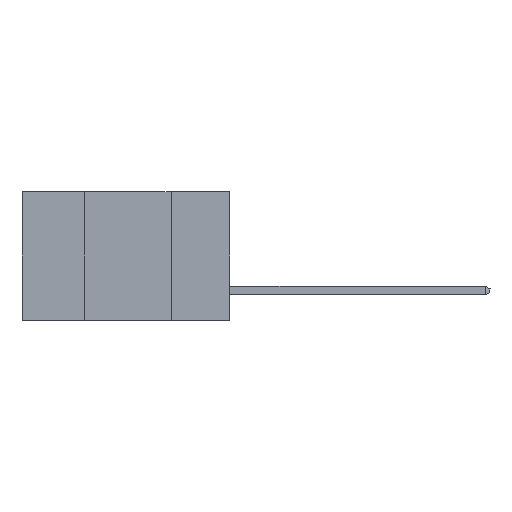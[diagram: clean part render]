
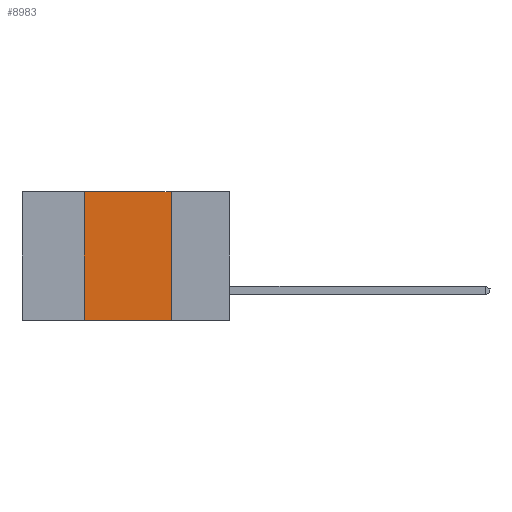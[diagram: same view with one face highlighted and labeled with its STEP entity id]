
A CAD part, left-side view. The second image highlights one B-rep face of the part: STEP entity #8983.
In plain terms, the highlighted planar face has unit normal (-1, 0, 0).
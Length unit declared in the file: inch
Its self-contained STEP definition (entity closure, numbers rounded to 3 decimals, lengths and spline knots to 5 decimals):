
#184 = VERTEX_POINT ( 'NONE', #4836 ) ;
#264 = EDGE_CURVE ( 'NONE', #184, #1446, #3708, .T. ) ;
#720 = DIRECTION ( 'NONE',  ( 0., -1., 0. ) ) ;
#741 = LINE ( 'NONE', #7236, #4051 ) ;
#1446 = VERTEX_POINT ( 'NONE', #8938 ) ;
#1547 = CARTESIAN_POINT ( 'NONE',  ( 0., 0.6, -0.37 ) ) ;
#1563 = VECTOR ( 'NONE', #4553, 39.37008 ) ;
#1700 = LINE ( 'NONE', #7397, #1563 ) ;
#1803 = DIRECTION ( 'NONE',  ( 1., 0., 0. ) ) ;
#2610 = ORIENTED_EDGE ( 'NONE', *, *, #6053, .F. ) ;
#2784 = VERTEX_POINT ( 'NONE', #3439 ) ;
#3439 = CARTESIAN_POINT ( 'NONE',  ( 0., 0.17, 0. ) ) ;
#3491 = CARTESIAN_POINT ( 'NONE',  ( 0., 0.6, 0. ) ) ;
#3534 = VECTOR ( 'NONE', #7159, 39.37008 ) ;
#3708 = LINE ( 'NONE', #1547, #3534 ) ;
#3890 = CARTESIAN_POINT ( 'NONE',  ( 0., 0.42, 0. ) ) ;
#4051 = VECTOR ( 'NONE', #8603, 39.37008 ) ;
#4087 = EDGE_CURVE ( 'NONE', #2784, #1446, #1700, .T. ) ;
#4553 = DIRECTION ( 'NONE',  ( 0., 0., -1. ) ) ;
#4580 = AXIS2_PLACEMENT_3D ( 'NONE', #4656, #1803, #5968 ) ;
#4656 = CARTESIAN_POINT ( 'NONE',  ( 0., 0.6, 0. ) ) ;
#4836 = CARTESIAN_POINT ( 'NONE',  ( 0., 0.42, -0.37 ) ) ;
#5589 = LINE ( 'NONE', #3491, #6911 ) ;
#5658 = ORIENTED_EDGE ( 'NONE', *, *, #6876, .F. ) ;
#5968 = DIRECTION ( 'NONE',  ( 0., 0., -1. ) ) ;
#6053 = EDGE_CURVE ( 'NONE', #184, #7036, #741, .T. ) ;
#6180 = ORIENTED_EDGE ( 'NONE', *, *, #4087, .F. ) ;
#6804 = EDGE_LOOP ( 'NONE', ( #6180, #5658, #2610, #8235 ) ) ;
#6876 = EDGE_CURVE ( 'NONE', #7036, #2784, #5589, .T. ) ;
#6911 = VECTOR ( 'NONE', #720, 39.37008 ) ;
#7036 = VERTEX_POINT ( 'NONE', #3890 ) ;
#7159 = DIRECTION ( 'NONE',  ( 0., -1., 0. ) ) ;
#7236 = CARTESIAN_POINT ( 'NONE',  ( 0., 0.42, -0.37 ) ) ;
#7397 = CARTESIAN_POINT ( 'NONE',  ( 0., 0.17, -0.37 ) ) ;
#8235 = ORIENTED_EDGE ( 'NONE', *, *, #264, .T. ) ;
#8603 = DIRECTION ( 'NONE',  ( 0., 0., 1. ) ) ;
#8814 = FACE_OUTER_BOUND ( 'NONE', #6804, .T. ) ;
#8865 = PLANE ( 'NONE',  #4580 ) ;
#8938 = CARTESIAN_POINT ( 'NONE',  ( 0., 0.17, -0.37 ) ) ;
#8983 = ADVANCED_FACE ( 'NONE', ( #8814 ), #8865, .F. ) ;
